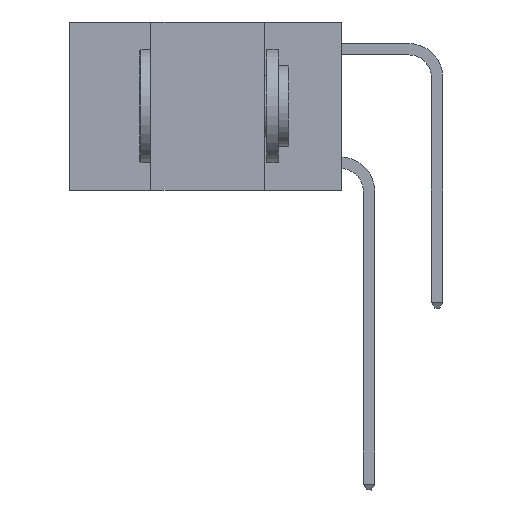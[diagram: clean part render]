
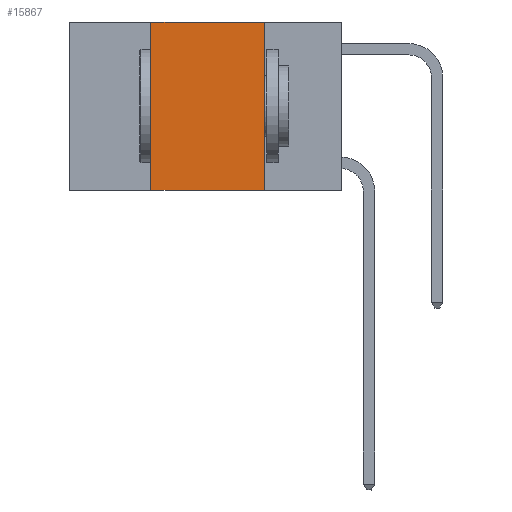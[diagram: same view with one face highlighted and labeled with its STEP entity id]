
A CAD part, left-side view. The second image highlights one B-rep face of the part: STEP entity #15867.
In plain terms, the highlighted planar face has unit normal (-1, 0, 0).
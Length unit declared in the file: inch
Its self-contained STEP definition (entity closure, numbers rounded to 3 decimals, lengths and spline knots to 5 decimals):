
#667 = LINE ( 'NONE', #18618, #11523 ) ;
#2169 = ORIENTED_EDGE ( 'NONE', *, *, #14007, .F. ) ;
#4395 = CARTESIAN_POINT ( 'NONE',  ( 0., 0.17, -0.37 ) ) ;
#4456 = EDGE_CURVE ( 'NONE', #13180, #23645, #667, .T. ) ;
#4792 = VECTOR ( 'NONE', #17936, 39.37008 ) ;
#6248 = CARTESIAN_POINT ( 'NONE',  ( 0., 0.6, 0. ) ) ;
#6798 = DIRECTION ( 'NONE',  ( 0., 0., 1. ) ) ;
#8305 = DIRECTION ( 'NONE',  ( 0., 0., -1. ) ) ;
#8375 = EDGE_LOOP ( 'NONE', ( #17010, #22078, #2169, #17618 ) ) ;
#8441 = DIRECTION ( 'NONE',  ( 0., 0., -1. ) ) ;
#9668 = VECTOR ( 'NONE', #8441, 39.37008 ) ;
#9975 = LINE ( 'NONE', #23558, #4792 ) ;
#10431 = CARTESIAN_POINT ( 'NONE',  ( 0., 0.17, 0. ) ) ;
#11090 = EDGE_CURVE ( 'NONE', #23645, #12218, #16087, .T. ) ;
#11523 = VECTOR ( 'NONE', #22422, 39.37008 ) ;
#12218 = VERTEX_POINT ( 'NONE', #4395 ) ;
#12529 = FACE_OUTER_BOUND ( 'NONE', #8375, .T. ) ;
#13180 = VERTEX_POINT ( 'NONE', #18089 ) ;
#14007 = EDGE_CURVE ( 'NONE', #17423, #13180, #23418, .T. ) ;
#14580 = CARTESIAN_POINT ( 'NONE',  ( 0., 0.42, -0.37 ) ) ;
#15867 = ADVANCED_FACE ( 'NONE', ( #12529 ), #16081, .F. ) ;
#16081 = PLANE ( 'NONE',  #19756 ) ;
#16087 = LINE ( 'NONE', #10431, #9668 ) ;
#17010 = ORIENTED_EDGE ( 'NONE', *, *, #11090, .F. ) ;
#17177 = VECTOR ( 'NONE', #6798, 39.37008 ) ;
#17423 = VERTEX_POINT ( 'NONE', #14580 ) ;
#17618 = ORIENTED_EDGE ( 'NONE', *, *, #21847, .T. ) ;
#17936 = DIRECTION ( 'NONE',  ( 0., -1., 0. ) ) ;
#18089 = CARTESIAN_POINT ( 'NONE',  ( 0., 0.42, 0. ) ) ;
#18618 = CARTESIAN_POINT ( 'NONE',  ( 0., 0.6, 0. ) ) ;
#19756 = AXIS2_PLACEMENT_3D ( 'NONE', #6248, #19933, #8305 ) ;
#19933 = DIRECTION ( 'NONE',  ( 1., 0., 0. ) ) ;
#21847 = EDGE_CURVE ( 'NONE', #17423, #12218, #9975, .T. ) ;
#22078 = ORIENTED_EDGE ( 'NONE', *, *, #4456, .F. ) ;
#22209 = CARTESIAN_POINT ( 'NONE',  ( 0., 0.42, 0. ) ) ;
#22422 = DIRECTION ( 'NONE',  ( 0., -1., 0. ) ) ;
#23418 = LINE ( 'NONE', #22209, #17177 ) ;
#23558 = CARTESIAN_POINT ( 'NONE',  ( 0., 0.6, -0.37 ) ) ;
#23564 = CARTESIAN_POINT ( 'NONE',  ( 0., 0.17, 0. ) ) ;
#23645 = VERTEX_POINT ( 'NONE', #23564 ) ;
